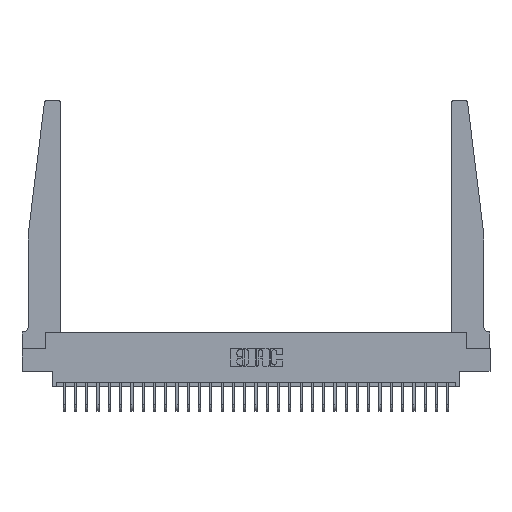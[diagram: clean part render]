
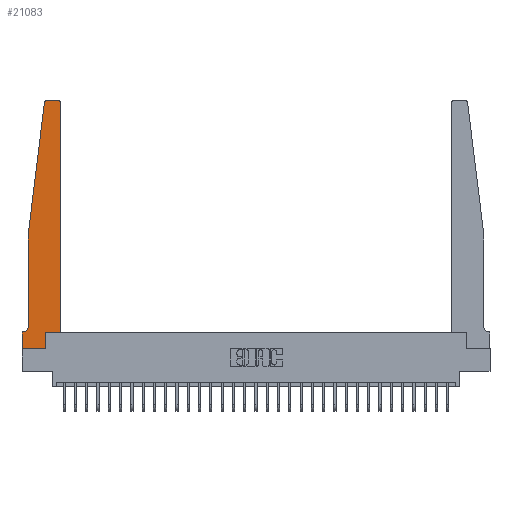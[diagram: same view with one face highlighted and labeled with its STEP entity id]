
A CAD part, top view. The second image highlights one B-rep face of the part: STEP entity #21083.
In plain terms, the highlighted planar face has unit normal (0, 0, 1).
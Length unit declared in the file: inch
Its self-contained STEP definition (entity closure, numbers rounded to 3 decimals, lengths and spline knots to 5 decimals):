
#935 = EDGE_CURVE ( 'NONE', #10780, #7217, #26731, .T. ) ;
#1217 = DIRECTION ( 'NONE',  ( 0., 1., 0. ) ) ;
#1279 = VECTOR ( 'NONE', #26287, 39.37008 ) ;
#1414 = CARTESIAN_POINT ( 'NONE',  ( 0.425, 2.72, 0.37 ) ) ;
#1601 = CARTESIAN_POINT ( 'NONE',  ( 0.25, 2.75, 0.37 ) ) ;
#1790 = VERTEX_POINT ( 'NONE', #11572 ) ;
#1826 = CARTESIAN_POINT ( 'NONE',  ( 0.395, 2.72, 0.37 ) ) ;
#2533 = EDGE_CURVE ( 'NONE', #19057, #5537, #13728, .T. ) ;
#2585 = VECTOR ( 'NONE', #24730, 39.37008 ) ;
#2666 = LINE ( 'NONE', #11328, #15022 ) ;
#2771 = CARTESIAN_POINT ( 'NONE',  ( 0.395, 2.75, 0.37 ) ) ;
#3144 = EDGE_CURVE ( 'NONE', #24927, #8599, #12663, .T. ) ;
#3184 = CARTESIAN_POINT ( 'NONE',  ( 0.425, 0.18, 0.37 ) ) ;
#3382 = EDGE_CURVE ( 'NONE', #26442, #12055, #9868, .T. ) ;
#3749 = ORIENTED_EDGE ( 'NONE', *, *, #4495, .T. ) ;
#3772 = ORIENTED_EDGE ( 'NONE', *, *, #935, .T. ) ;
#3788 = ORIENTED_EDGE ( 'NONE', *, *, #20501, .T. ) ;
#4226 = VECTOR ( 'NONE', #10175, 39.37008 ) ;
#4393 = LINE ( 'NONE', #6670, #1279 ) ;
#4495 = EDGE_CURVE ( 'NONE', #7217, #1790, #4393, .T. ) ;
#5245 = CARTESIAN_POINT ( 'NONE',  ( 0., 0., 0.37 ) ) ;
#5376 = EDGE_CURVE ( 'NONE', #24621, #10780, #14094, .T. ) ;
#5537 = VERTEX_POINT ( 'NONE', #28011 ) ;
#5852 = CARTESIAN_POINT ( 'NONE',  ( 0., 0.1875, 0.37 ) ) ;
#6259 = CARTESIAN_POINT ( 'NONE',  ( 0.2605, 0.18, 0.37 ) ) ;
#6615 = ORIENTED_EDGE ( 'NONE', *, *, #22697, .T. ) ;
#6670 = CARTESIAN_POINT ( 'NONE',  ( 0.065, 1.25, 0.37 ) ) ;
#6962 = AXIS2_PLACEMENT_3D ( 'NONE', #5852, #16464, #21452 ) ;
#7217 = VERTEX_POINT ( 'NONE', #8108 ) ;
#7350 = CARTESIAN_POINT ( 'NONE',  ( 0., 0.1875, 0.37 ) ) ;
#7618 = ORIENTED_EDGE ( 'NONE', *, *, #5376, .T. ) ;
#8108 = CARTESIAN_POINT ( 'NONE',  ( 0.24675, 2.72367, 0.37 ) ) ;
#8599 = VERTEX_POINT ( 'NONE', #6259 ) ;
#8804 = CARTESIAN_POINT ( 'NONE',  ( 0.015, 0.1875, 0.37 ) ) ;
#9868 = CIRCLE ( 'NONE', #20292, 0.05 ) ;
#10148 = DIRECTION ( 'NONE',  ( 0., 0., -1. ) ) ;
#10175 = DIRECTION ( 'NONE',  ( 0., -1., 0. ) ) ;
#10255 = VECTOR ( 'NONE', #1217, 39.37008 ) ;
#10780 = VERTEX_POINT ( 'NONE', #23633 ) ;
#10806 = ORIENTED_EDGE ( 'NONE', *, *, #20771, .T. ) ;
#11200 = LINE ( 'NONE', #5245, #15076 ) ;
#11328 = CARTESIAN_POINT ( 'NONE',  ( 0.065, 0.1875, 0.37 ) ) ;
#11572 = CARTESIAN_POINT ( 'NONE',  ( 0.065, 1.25, 0.37 ) ) ;
#12055 = VERTEX_POINT ( 'NONE', #8804 ) ;
#12342 = FACE_OUTER_BOUND ( 'NONE', #19464, .T. ) ;
#12663 = LINE ( 'NONE', #19194, #14135 ) ;
#12730 = DIRECTION ( 'NONE',  ( 0., 0., 1. ) ) ;
#12738 = PLANE ( 'NONE',  #6962 ) ;
#13606 = DIRECTION ( 'NONE',  ( 1., 0., 0. ) ) ;
#13673 = CARTESIAN_POINT ( 'NONE',  ( 0.065, 0.2375, 0.37 ) ) ;
#13728 = LINE ( 'NONE', #16005, #2585 ) ;
#14094 = LINE ( 'NONE', #1601, #27708 ) ;
#14106 = VERTEX_POINT ( 'NONE', #26679 ) ;
#14135 = VECTOR ( 'NONE', #17723, 39.37008 ) ;
#14293 = AXIS2_PLACEMENT_3D ( 'NONE', #1826, #12730, #19407 ) ;
#14446 = AXIS2_PLACEMENT_3D ( 'NONE', #17753, #21919, #15769 ) ;
#15022 = VECTOR ( 'NONE', #15988, 39.37008 ) ;
#15076 = VECTOR ( 'NONE', #13606, 39.37008 ) ;
#15769 = DIRECTION ( 'NONE',  ( 1., 0., 0. ) ) ;
#15919 = ORIENTED_EDGE ( 'NONE', *, *, #24341, .T. ) ;
#15988 = DIRECTION ( 'NONE',  ( -1., 0., 0. ) ) ;
#16005 = CARTESIAN_POINT ( 'NONE',  ( 0., 0., 0.37 ) ) ;
#16247 = DIRECTION ( 'NONE',  ( -1., 0., 0. ) ) ;
#16464 = DIRECTION ( 'NONE',  ( 0., 0., 1. ) ) ;
#17430 = VERTEX_POINT ( 'NONE', #1414 ) ;
#17723 = DIRECTION ( 'NONE',  ( 0., 1., 0. ) ) ;
#17753 = CARTESIAN_POINT ( 'NONE',  ( 0.27653, 2.72, 0.37 ) ) ;
#18333 = DIRECTION ( 'NONE',  ( 1., 0., 0. ) ) ;
#18345 = ORIENTED_EDGE ( 'NONE', *, *, #2533, .T. ) ;
#18635 = DIRECTION ( 'NONE',  ( -1., 0., 0. ) ) ;
#19057 = VERTEX_POINT ( 'NONE', #7350 ) ;
#19194 = CARTESIAN_POINT ( 'NONE',  ( 0.2605, 0.18, 0.37 ) ) ;
#19407 = DIRECTION ( 'NONE',  ( 1., 0., 0. ) ) ;
#19459 = ORIENTED_EDGE ( 'NONE', *, *, #3144, .T. ) ;
#19464 = EDGE_LOOP ( 'NONE', ( #7618, #3772, #3749, #15919, #27330, #3788, #18345, #6615, #19459, #10806, #22098, #23592 ) ) ;
#19550 = VECTOR ( 'NONE', #18333, 39.37008 ) ;
#20292 = AXIS2_PLACEMENT_3D ( 'NONE', #20814, #10148, #16247 ) ;
#20393 = LINE ( 'NONE', #22818, #10255 ) ;
#20501 = EDGE_CURVE ( 'NONE', #12055, #19057, #2666, .T. ) ;
#20771 = EDGE_CURVE ( 'NONE', #8599, #14106, #26787, .T. ) ;
#20814 = CARTESIAN_POINT ( 'NONE',  ( 0.015, 0.2375, 0.37 ) ) ;
#21083 = ADVANCED_FACE ( 'NONE', ( #12342 ), #12738, .T. ) ;
#21452 = DIRECTION ( 'NONE',  ( 1., 0., 0. ) ) ;
#21919 = DIRECTION ( 'NONE',  ( 0., 0., 1. ) ) ;
#22098 = ORIENTED_EDGE ( 'NONE', *, *, #27276, .T. ) ;
#22634 = CARTESIAN_POINT ( 'NONE',  ( 0.2605, 0., 0.37 ) ) ;
#22697 = EDGE_CURVE ( 'NONE', #5537, #24927, #11200, .T. ) ;
#22818 = CARTESIAN_POINT ( 'NONE',  ( 0.425, 0.18, 0.37 ) ) ;
#23117 = LINE ( 'NONE', #27267, #4226 ) ;
#23592 = ORIENTED_EDGE ( 'NONE', *, *, #26868, .T. ) ;
#23633 = CARTESIAN_POINT ( 'NONE',  ( 0.27653, 2.75, 0.37 ) ) ;
#24341 = EDGE_CURVE ( 'NONE', #1790, #26442, #23117, .T. ) ;
#24621 = VERTEX_POINT ( 'NONE', #2771 ) ;
#24730 = DIRECTION ( 'NONE',  ( 0., -1., 0. ) ) ;
#24777 = CIRCLE ( 'NONE', #14293, 0.03 ) ;
#24927 = VERTEX_POINT ( 'NONE', #22634 ) ;
#26287 = DIRECTION ( 'NONE',  ( -0.122, -0.992, 0. ) ) ;
#26442 = VERTEX_POINT ( 'NONE', #13673 ) ;
#26679 = CARTESIAN_POINT ( 'NONE',  ( 0.425, 0.18, 0.37 ) ) ;
#26731 = CIRCLE ( 'NONE', #14446, 0.03 ) ;
#26787 = LINE ( 'NONE', #3184, #19550 ) ;
#26868 = EDGE_CURVE ( 'NONE', #17430, #24621, #24777, .T. ) ;
#27267 = CARTESIAN_POINT ( 'NONE',  ( 0.065, 1.25, 0.37 ) ) ;
#27276 = EDGE_CURVE ( 'NONE', #14106, #17430, #20393, .T. ) ;
#27330 = ORIENTED_EDGE ( 'NONE', *, *, #3382, .T. ) ;
#27708 = VECTOR ( 'NONE', #18635, 39.37008 ) ;
#28011 = CARTESIAN_POINT ( 'NONE',  ( 0., 0., 0.37 ) ) ;
